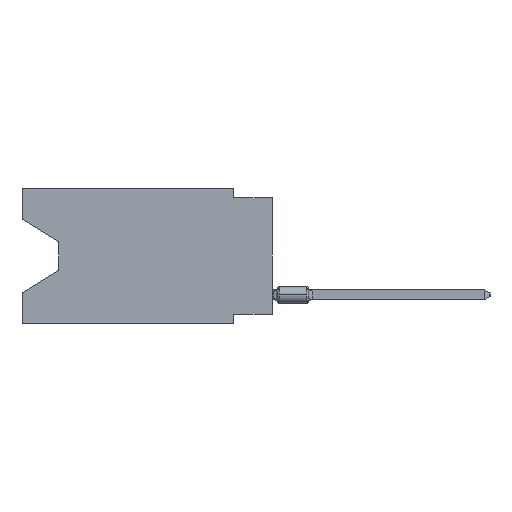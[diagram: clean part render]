
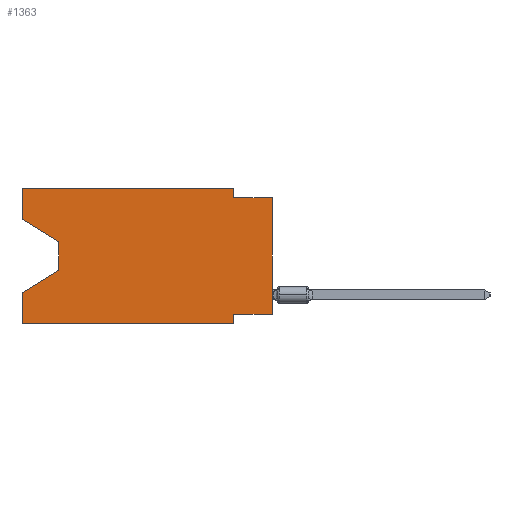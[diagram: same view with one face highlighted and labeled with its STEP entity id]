
A CAD part, left-side view. The second image highlights one B-rep face of the part: STEP entity #1363.
In plain terms, the highlighted planar face has unit normal (-1, 0, 0).
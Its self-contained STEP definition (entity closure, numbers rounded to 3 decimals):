
#487 = LINE ( 'NONE', #22792, #49641 ) ;
#699 = DIRECTION ( 'NONE',  ( 0., 0., -1. ) ) ;
#826 = VERTEX_POINT ( 'NONE', #9402 ) ;
#976 = ORIENTED_EDGE ( 'NONE', *, *, #62939, .F. ) ;
#1081 = CARTESIAN_POINT ( 'NONE',  ( 0., 16.383, -2.038 ) ) ;
#1171 = CARTESIAN_POINT ( 'NONE',  ( 0., 0., -0.635 ) ) ;
#1363 = ADVANCED_FACE ( 'NONE', ( #22369 ), #33703, .F. ) ;
#1438 = DIRECTION ( 'NONE',  ( 0., -1., 0. ) ) ;
#2082 = VECTOR ( 'NONE', #1438, 1000. ) ;
#2924 = ORIENTED_EDGE ( 'NONE', *, *, #20273, .F. ) ;
#4931 = CARTESIAN_POINT ( 'NONE',  ( 0., 13.97, -3.505 ) ) ;
#4980 = ORIENTED_EDGE ( 'NONE', *, *, #61764, .T. ) ;
#5090 = EDGE_LOOP ( 'NONE', ( #23651, #32126, #4980, #24802, #45543, #33707, #53871, #58764, #976, #70888, #2924, #10816 ) ) ;
#5170 = LINE ( 'NONE', #43546, #8064 ) ;
#5322 = EDGE_CURVE ( 'NONE', #63293, #62423, #20685, .T. ) ;
#5555 = VERTEX_POINT ( 'NONE', #53645 ) ;
#7786 = VERTEX_POINT ( 'NONE', #28551 ) ;
#8064 = VECTOR ( 'NONE', #49018, 1000. ) ;
#9358 = DIRECTION ( 'NONE',  ( 0., -0.855, -0.519 ) ) ;
#9402 = CARTESIAN_POINT ( 'NONE',  ( 0., 16.383, -8.89 ) ) ;
#10816 = ORIENTED_EDGE ( 'NONE', *, *, #13794, .F. ) ;
#11753 = CARTESIAN_POINT ( 'NONE',  ( 0., 0., 0. ) ) ;
#13794 = EDGE_CURVE ( 'NONE', #63293, #49035, #43876, .T. ) ;
#16925 = DIRECTION ( 'NONE',  ( 0., 0., -1. ) ) ;
#17135 = VERTEX_POINT ( 'NONE', #68228 ) ;
#18301 = VERTEX_POINT ( 'NONE', #38473 ) ;
#20273 = EDGE_CURVE ( 'NONE', #49035, #5555, #45649, .T. ) ;
#20685 = LINE ( 'NONE', #63828, #24624 ) ;
#22120 = CARTESIAN_POINT ( 'NONE',  ( 0., 13.97, -5.385 ) ) ;
#22294 = CARTESIAN_POINT ( 'NONE',  ( 0., 0., -0.635 ) ) ;
#22369 = FACE_OUTER_BOUND ( 'NONE', #5090, .T. ) ;
#22792 = CARTESIAN_POINT ( 'NONE',  ( 0., 16.383, -8.89 ) ) ;
#23651 = ORIENTED_EDGE ( 'NONE', *, *, #5322, .T. ) ;
#23815 = DIRECTION ( 'NONE',  ( 1., 0., 0. ) ) ;
#24624 = VECTOR ( 'NONE', #9358, 1000. ) ;
#24802 = ORIENTED_EDGE ( 'NONE', *, *, #54260, .F. ) ;
#28551 = CARTESIAN_POINT ( 'NONE',  ( 0., 0., -8.255 ) ) ;
#28554 = DIRECTION ( 'NONE',  ( 0., 0., -1. ) ) ;
#28681 = CARTESIAN_POINT ( 'NONE',  ( 0., 2.54, -0.635 ) ) ;
#28903 = DIRECTION ( 'NONE',  ( 0., 0., 1. ) ) ;
#29914 = VERTEX_POINT ( 'NONE', #22120 ) ;
#31524 = EDGE_CURVE ( 'NONE', #7786, #62163, #61809, .T. ) ;
#32126 = ORIENTED_EDGE ( 'NONE', *, *, #63407, .T. ) ;
#32881 = VECTOR ( 'NONE', #60802, 1000. ) ;
#33631 = VECTOR ( 'NONE', #16925, 1000. ) ;
#33703 = PLANE ( 'NONE',  #40626 ) ;
#33707 = ORIENTED_EDGE ( 'NONE', *, *, #64391, .F. ) ;
#34053 = DIRECTION ( 'NONE',  ( 0., 0., 1. ) ) ;
#34701 = CARTESIAN_POINT ( 'NONE',  ( 0., 16.383, 0. ) ) ;
#35127 = CARTESIAN_POINT ( 'NONE',  ( 0., 16.383, 0. ) ) ;
#36251 = EDGE_CURVE ( 'NONE', #7786, #62925, #5170, .T. ) ;
#38473 = CARTESIAN_POINT ( 'NONE',  ( 0., 2.54, -8.89 ) ) ;
#38528 = CARTESIAN_POINT ( 'NONE',  ( 0., 2.54, 0. ) ) ;
#39175 = LINE ( 'NONE', #1171, #50904 ) ;
#39344 = VECTOR ( 'NONE', #699, 1000. ) ;
#40200 = LINE ( 'NONE', #40564, #63230 ) ;
#40564 = CARTESIAN_POINT ( 'NONE',  ( 0., 16.383, 0. ) ) ;
#40626 = AXIS2_PLACEMENT_3D ( 'NONE', #55955, #23815, #28554 ) ;
#43546 = CARTESIAN_POINT ( 'NONE',  ( 0., 0., -8.255 ) ) ;
#43876 = LINE ( 'NONE', #35127, #60891 ) ;
#43981 = LINE ( 'NONE', #38528, #32881 ) ;
#44287 = CARTESIAN_POINT ( 'NONE',  ( 0., 13.97, -5.385 ) ) ;
#45543 = ORIENTED_EDGE ( 'NONE', *, *, #60036, .T. ) ;
#45649 = LINE ( 'NONE', #34701, #2082 ) ;
#49018 = DIRECTION ( 'NONE',  ( 0., 1., 0. ) ) ;
#49035 = VERTEX_POINT ( 'NONE', #63732 ) ;
#49067 = CARTESIAN_POINT ( 'NONE',  ( 0., 2.54, -8.89 ) ) ;
#49641 = VECTOR ( 'NONE', #51276, 1000. ) ;
#50756 = CARTESIAN_POINT ( 'NONE',  ( 0., 13.97, -3.505 ) ) ;
#50904 = VECTOR ( 'NONE', #66595, 1000. ) ;
#51222 = CARTESIAN_POINT ( 'NONE',  ( 0., 2.54, -8.255 ) ) ;
#51276 = DIRECTION ( 'NONE',  ( 0., -1., 0. ) ) ;
#52143 = VECTOR ( 'NONE', #34053, 1000. ) ;
#53645 = CARTESIAN_POINT ( 'NONE',  ( 0., 2.54, 0. ) ) ;
#53871 = ORIENTED_EDGE ( 'NONE', *, *, #36251, .F. ) ;
#54083 = EDGE_CURVE ( 'NONE', #5555, #64013, #43981, .T. ) ;
#54260 = EDGE_CURVE ( 'NONE', #826, #17135, #40200, .T. ) ;
#55166 = LINE ( 'NONE', #50756, #39344 ) ;
#55242 = LINE ( 'NONE', #44287, #57853 ) ;
#55955 = CARTESIAN_POINT ( 'NONE',  ( 0., 16.383, 0. ) ) ;
#57853 = VECTOR ( 'NONE', #66579, 1000. ) ;
#58764 = ORIENTED_EDGE ( 'NONE', *, *, #31524, .T. ) ;
#60036 = EDGE_CURVE ( 'NONE', #826, #18301, #487, .T. ) ;
#60802 = DIRECTION ( 'NONE',  ( 0., 0., -1. ) ) ;
#60891 = VECTOR ( 'NONE', #28903, 1000. ) ;
#61764 = EDGE_CURVE ( 'NONE', #29914, #17135, #55242, .T. ) ;
#61809 = LINE ( 'NONE', #11753, #52143 ) ;
#62163 = VERTEX_POINT ( 'NONE', #22294 ) ;
#62423 = VERTEX_POINT ( 'NONE', #4931 ) ;
#62925 = VERTEX_POINT ( 'NONE', #51222 ) ;
#62939 = EDGE_CURVE ( 'NONE', #64013, #62163, #39175, .T. ) ;
#63230 = VECTOR ( 'NONE', #64557, 1000. ) ;
#63293 = VERTEX_POINT ( 'NONE', #1081 ) ;
#63407 = EDGE_CURVE ( 'NONE', #62423, #29914, #55166, .T. ) ;
#63732 = CARTESIAN_POINT ( 'NONE',  ( 0., 16.383, 0. ) ) ;
#63828 = CARTESIAN_POINT ( 'NONE',  ( 0., 16.383, -2.038 ) ) ;
#64013 = VERTEX_POINT ( 'NONE', #28681 ) ;
#64391 = EDGE_CURVE ( 'NONE', #62925, #18301, #65882, .T. ) ;
#64557 = DIRECTION ( 'NONE',  ( 0., 0., 1. ) ) ;
#65882 = LINE ( 'NONE', #49067, #33631 ) ;
#66579 = DIRECTION ( 'NONE',  ( 0., 0.855, -0.519 ) ) ;
#66595 = DIRECTION ( 'NONE',  ( 0., -1., 0. ) ) ;
#68228 = CARTESIAN_POINT ( 'NONE',  ( 0., 16.383, -6.852 ) ) ;
#70888 = ORIENTED_EDGE ( 'NONE', *, *, #54083, .F. ) ;
